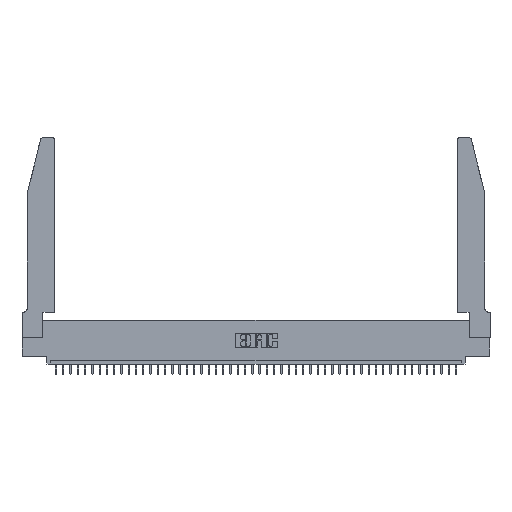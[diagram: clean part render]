
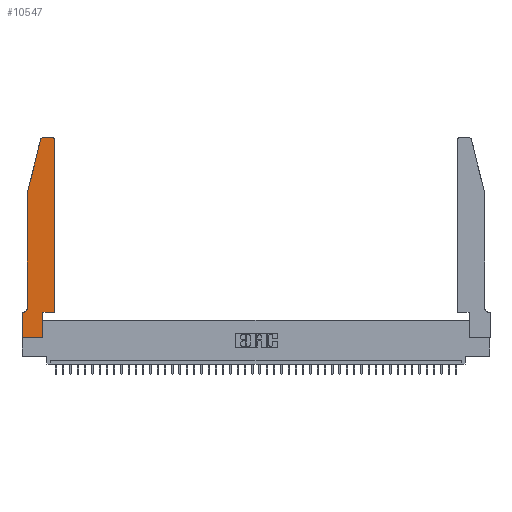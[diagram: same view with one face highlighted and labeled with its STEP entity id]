
A CAD part, top view. The second image highlights one B-rep face of the part: STEP entity #10547.
In plain terms, the highlighted planar face has unit normal (0, 0, 1).
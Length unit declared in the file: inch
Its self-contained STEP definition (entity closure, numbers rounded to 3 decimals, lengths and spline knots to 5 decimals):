
#110 = ORIENTED_EDGE ( 'NONE', *, *, #9006, .T. ) ;
#971 = EDGE_CURVE ( 'NONE', #16248, #44628, #2963, .T. ) ;
#974 = CIRCLE ( 'NONE', #31042, 0.03 ) ;
#1219 = LINE ( 'NONE', #22299, #30717 ) ;
#1934 = EDGE_CURVE ( 'NONE', #2622, #14081, #11076, .T. ) ;
#1988 = AXIS2_PLACEMENT_3D ( 'NONE', #24660, #18024, #13887 ) ;
#1991 = LINE ( 'NONE', #15976, #10499 ) ;
#2126 = EDGE_CURVE ( 'NONE', #30424, #12299, #1219, .T. ) ;
#2175 = DIRECTION ( 'NONE',  ( 1., 0., 0. ) ) ;
#2622 = VERTEX_POINT ( 'NONE', #16289 ) ;
#2918 = CARTESIAN_POINT ( 'NONE',  ( 0.0055, 0.35, 0.37 ) ) ;
#2951 = CARTESIAN_POINT ( 'NONE',  ( 0.4505, 2.72, 0.37 ) ) ;
#2963 = LINE ( 'NONE', #19950, #24748 ) ;
#3359 = CARTESIAN_POINT ( 'NONE',  ( 0.4505, 0.35, 0.37 ) ) ;
#4226 = CARTESIAN_POINT ( 'NONE',  ( 0.0755, 2., 0.37 ) ) ;
#4422 = AXIS2_PLACEMENT_3D ( 'NONE', #34033, #9272, #20276 ) ;
#5863 = DIRECTION ( 'NONE',  ( 1., 0., 0. ) ) ;
#6100 = CARTESIAN_POINT ( 'NONE',  ( 0.4205, 2.75, 0.37 ) ) ;
#6600 = VECTOR ( 'NONE', #9258, 39.37008 ) ;
#6761 = ORIENTED_EDGE ( 'NONE', *, *, #32200, .T. ) ;
#8383 = EDGE_CURVE ( 'NONE', #40313, #35130, #25914, .T. ) ;
#9006 = EDGE_CURVE ( 'NONE', #35130, #30424, #15900, .T. ) ;
#9046 = VECTOR ( 'NONE', #39373, 39.37008 ) ;
#9258 = DIRECTION ( 'NONE',  ( -1., 0., 0. ) ) ;
#9272 = DIRECTION ( 'NONE',  ( 0., 0., -1. ) ) ;
#9299 = AXIS2_PLACEMENT_3D ( 'NONE', #33569, #12493, #2175 ) ;
#9370 = ORIENTED_EDGE ( 'NONE', *, *, #12943, .T. ) ;
#9731 = VECTOR ( 'NONE', #27391, 39.37008 ) ;
#10488 = CARTESIAN_POINT ( 'NONE',  ( 0.4205, 2.72, 0.37 ) ) ;
#10499 = VECTOR ( 'NONE', #5863, 39.37008 ) ;
#10547 = ADVANCED_FACE ( 'NONE', ( #44055 ), #13170, .T. ) ;
#11076 = LINE ( 'NONE', #21402, #14587 ) ;
#11385 = DIRECTION ( 'NONE',  ( 1., 0., 0. ) ) ;
#12299 = VERTEX_POINT ( 'NONE', #21286 ) ;
#12493 = DIRECTION ( 'NONE',  ( 0., 0., 1. ) ) ;
#12720 = LINE ( 'NONE', #43367, #35404 ) ;
#12943 = EDGE_CURVE ( 'NONE', #20789, #17830, #24196, .T. ) ;
#13079 = ORIENTED_EDGE ( 'NONE', *, *, #971, .T. ) ;
#13170 = PLANE ( 'NONE',  #9299 ) ;
#13475 = VERTEX_POINT ( 'NONE', #41255 ) ;
#13506 = DIRECTION ( 'NONE',  ( 0., 1., 0. ) ) ;
#13693 = CARTESIAN_POINT ( 'NONE',  ( 0.2865, 0., 0.37 ) ) ;
#13887 = DIRECTION ( 'NONE',  ( 1., 0., 0. ) ) ;
#14081 = VERTEX_POINT ( 'NONE', #39337 ) ;
#14587 = VECTOR ( 'NONE', #41742, 39.37008 ) ;
#14834 = ORIENTED_EDGE ( 'NONE', *, *, #25111, .T. ) ;
#15642 = VERTEX_POINT ( 'NONE', #13693 ) ;
#15900 = CIRCLE ( 'NONE', #1988, 0.03 ) ;
#15976 = CARTESIAN_POINT ( 'NONE',  ( 0.4505, 0.35, 0.37 ) ) ;
#16248 = VERTEX_POINT ( 'NONE', #3359 ) ;
#16289 = CARTESIAN_POINT ( 'NONE',  ( 0., 0.35, 0.37 ) ) ;
#16567 = EDGE_CURVE ( 'NONE', #15642, #13475, #37198, .T. ) ;
#16813 = EDGE_LOOP ( 'NONE', ( #41787, #110, #39284, #29604, #9370, #6761, #32597, #23365, #20564, #14834, #13079, #22586 ) ) ;
#17830 = VERTEX_POINT ( 'NONE', #2918 ) ;
#18024 = DIRECTION ( 'NONE',  ( 0., 0., 1. ) ) ;
#18481 = DIRECTION ( 'NONE',  ( 0., -1., 0. ) ) ;
#18544 = CARTESIAN_POINT ( 'NONE',  ( 0.284, 2.75, 0.37 ) ) ;
#19950 = CARTESIAN_POINT ( 'NONE',  ( 0.4505, 0.35, 0.37 ) ) ;
#20276 = DIRECTION ( 'NONE',  ( -1., 0., 0. ) ) ;
#20564 = ORIENTED_EDGE ( 'NONE', *, *, #16567, .T. ) ;
#20677 = EDGE_CURVE ( 'NONE', #12299, #20789, #32452, .T. ) ;
#20789 = VERTEX_POINT ( 'NONE', #39724 ) ;
#21286 = CARTESIAN_POINT ( 'NONE',  ( 0.0755, 2., 0.37 ) ) ;
#21402 = CARTESIAN_POINT ( 'NONE',  ( 0., 0., 0.37 ) ) ;
#22299 = CARTESIAN_POINT ( 'NONE',  ( 0.0755, 2., 0.37 ) ) ;
#22586 = ORIENTED_EDGE ( 'NONE', *, *, #37514, .T. ) ;
#23365 = ORIENTED_EDGE ( 'NONE', *, *, #25501, .T. ) ;
#24196 = CIRCLE ( 'NONE', #4422, 0.07 ) ;
#24660 = CARTESIAN_POINT ( 'NONE',  ( 0.284, 2.72, 0.37 ) ) ;
#24748 = VECTOR ( 'NONE', #13506, 39.37008 ) ;
#25111 = EDGE_CURVE ( 'NONE', #13475, #16248, #1991, .T. ) ;
#25501 = EDGE_CURVE ( 'NONE', #14081, #15642, #12720, .T. ) ;
#25914 = LINE ( 'NONE', #39842, #9046 ) ;
#26017 = DIRECTION ( 'NONE',  ( 1., 0., 0. ) ) ;
#27391 = DIRECTION ( 'NONE',  ( 0., 1., 0. ) ) ;
#27818 = CARTESIAN_POINT ( 'NONE',  ( 0.0755, 0.35, 0.37 ) ) ;
#29432 = DIRECTION ( 'NONE',  ( -0.239, -0.971, 0. ) ) ;
#29604 = ORIENTED_EDGE ( 'NONE', *, *, #20677, .T. ) ;
#30424 = VERTEX_POINT ( 'NONE', #40642 ) ;
#30717 = VECTOR ( 'NONE', #29432, 39.37008 ) ;
#31042 = AXIS2_PLACEMENT_3D ( 'NONE', #10488, #32030, #11385 ) ;
#32030 = DIRECTION ( 'NONE',  ( 0., 0., 1. ) ) ;
#32162 = VECTOR ( 'NONE', #18481, 39.37008 ) ;
#32200 = EDGE_CURVE ( 'NONE', #17830, #2622, #45158, .T. ) ;
#32452 = LINE ( 'NONE', #4226, #32162 ) ;
#32597 = ORIENTED_EDGE ( 'NONE', *, *, #1934, .T. ) ;
#33569 = CARTESIAN_POINT ( 'NONE',  ( 0., 0.35, 0.37 ) ) ;
#34027 = CARTESIAN_POINT ( 'NONE',  ( 0.2865, 0.35, 0.37 ) ) ;
#34033 = CARTESIAN_POINT ( 'NONE',  ( 0.0055, 0.42, 0.37 ) ) ;
#35130 = VERTEX_POINT ( 'NONE', #18544 ) ;
#35404 = VECTOR ( 'NONE', #26017, 39.37008 ) ;
#37198 = LINE ( 'NONE', #34027, #9731 ) ;
#37514 = EDGE_CURVE ( 'NONE', #44628, #40313, #974, .T. ) ;
#39284 = ORIENTED_EDGE ( 'NONE', *, *, #2126, .T. ) ;
#39337 = CARTESIAN_POINT ( 'NONE',  ( 0., 0., 0.37 ) ) ;
#39373 = DIRECTION ( 'NONE',  ( -1., 0., 0. ) ) ;
#39724 = CARTESIAN_POINT ( 'NONE',  ( 0.0755, 0.42, 0.37 ) ) ;
#39842 = CARTESIAN_POINT ( 'NONE',  ( 0.2605, 2.75, 0.37 ) ) ;
#40313 = VERTEX_POINT ( 'NONE', #6100 ) ;
#40642 = CARTESIAN_POINT ( 'NONE',  ( 0.25487, 2.72718, 0.37 ) ) ;
#41255 = CARTESIAN_POINT ( 'NONE',  ( 0.2865, 0.35, 0.37 ) ) ;
#41742 = DIRECTION ( 'NONE',  ( 0., -1., 0. ) ) ;
#41787 = ORIENTED_EDGE ( 'NONE', *, *, #8383, .T. ) ;
#43367 = CARTESIAN_POINT ( 'NONE',  ( 0., 0., 0.37 ) ) ;
#44055 = FACE_OUTER_BOUND ( 'NONE', #16813, .T. ) ;
#44628 = VERTEX_POINT ( 'NONE', #2951 ) ;
#45158 = LINE ( 'NONE', #27818, #6600 ) ;
